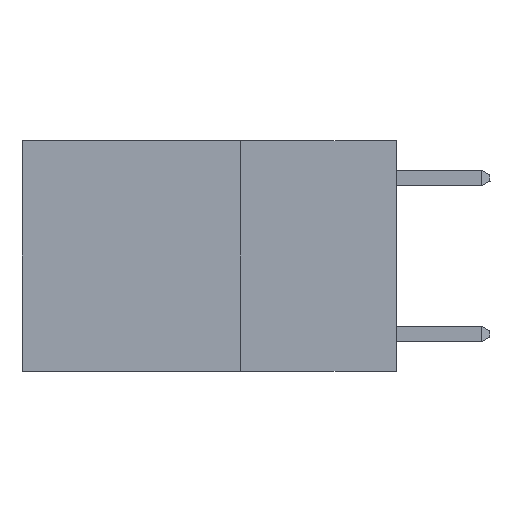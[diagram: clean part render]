
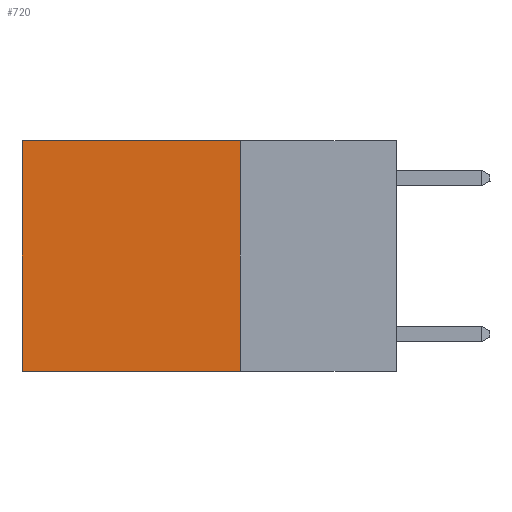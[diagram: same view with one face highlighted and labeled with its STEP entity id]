
A CAD part, left-side view. The second image highlights one B-rep face of the part: STEP entity #720.
In plain terms, the highlighted planar face has unit normal (-1, 0, 0).
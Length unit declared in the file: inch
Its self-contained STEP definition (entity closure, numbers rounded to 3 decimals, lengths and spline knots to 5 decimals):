
#720 = ADVANCED_FACE ( 'NONE', ( #5217 ), #2796, .F. ) ;
#1088 = DIRECTION ( 'NONE',  ( 0., 0., -1. ) ) ;
#1827 = VERTEX_POINT ( 'NONE', #3212 ) ;
#1837 = ORIENTED_EDGE ( 'NONE', *, *, #3436, .T. ) ;
#2602 = EDGE_CURVE ( 'NONE', #1827, #11287, #8816, .T. ) ;
#2796 = PLANE ( 'NONE',  #6064 ) ;
#2925 = CARTESIAN_POINT ( 'NONE',  ( 0.2625, 0.25, 0. ) ) ;
#2936 = ORIENTED_EDGE ( 'NONE', *, *, #3915, .T. ) ;
#2951 = VECTOR ( 'NONE', #4636, 39.37008 ) ;
#2998 = DIRECTION ( 'NONE',  ( 0., 1., 0. ) ) ;
#3212 = CARTESIAN_POINT ( 'NONE',  ( 0.2625, 0.25, 0. ) ) ;
#3436 = EDGE_CURVE ( 'NONE', #10691, #11419, #9345, .T. ) ;
#3729 = CARTESIAN_POINT ( 'NONE',  ( 0.2625, 0.25, -0.37 ) ) ;
#3903 = CARTESIAN_POINT ( 'NONE',  ( 0.2625, 0.6, -0.37 ) ) ;
#3915 = EDGE_CURVE ( 'NONE', #1827, #10691, #7742, .T. ) ;
#4197 = VECTOR ( 'NONE', #1088, 39.37008 ) ;
#4636 = DIRECTION ( 'NONE',  ( 0., 1., 0. ) ) ;
#5217 = FACE_OUTER_BOUND ( 'NONE', #10482, .T. ) ;
#5576 = DIRECTION ( 'NONE',  ( 0., 0., -1. ) ) ;
#5638 = DIRECTION ( 'NONE',  ( 1., 0., 0. ) ) ;
#6064 = AXIS2_PLACEMENT_3D ( 'NONE', #9054, #5638, #7101 ) ;
#6111 = ORIENTED_EDGE ( 'NONE', *, *, #8259, .F. ) ;
#6996 = VECTOR ( 'NONE', #5576, 39.37008 ) ;
#7101 = DIRECTION ( 'NONE',  ( 0., 0., -1. ) ) ;
#7320 = CARTESIAN_POINT ( 'NONE',  ( 0.2625, 0.25, -0.37 ) ) ;
#7442 = CARTESIAN_POINT ( 'NONE',  ( 0.2625, 0.6, 0. ) ) ;
#7742 = LINE ( 'NONE', #2925, #8664 ) ;
#7989 = CARTESIAN_POINT ( 'NONE',  ( 0.2625, 0.25, 0. ) ) ;
#8259 = EDGE_CURVE ( 'NONE', #11287, #11419, #9109, .T. ) ;
#8664 = VECTOR ( 'NONE', #2998, 39.37008 ) ;
#8816 = LINE ( 'NONE', #7989, #4197 ) ;
#9054 = CARTESIAN_POINT ( 'NONE',  ( 0.2625, 0.25, 0. ) ) ;
#9109 = LINE ( 'NONE', #3729, #2951 ) ;
#9345 = LINE ( 'NONE', #7442, #6996 ) ;
#10482 = EDGE_LOOP ( 'NONE', ( #1837, #6111, #10554, #2936 ) ) ;
#10554 = ORIENTED_EDGE ( 'NONE', *, *, #2602, .F. ) ;
#10691 = VERTEX_POINT ( 'NONE', #10841 ) ;
#10841 = CARTESIAN_POINT ( 'NONE',  ( 0.2625, 0.6, 0. ) ) ;
#11287 = VERTEX_POINT ( 'NONE', #7320 ) ;
#11419 = VERTEX_POINT ( 'NONE', #3903 ) ;
